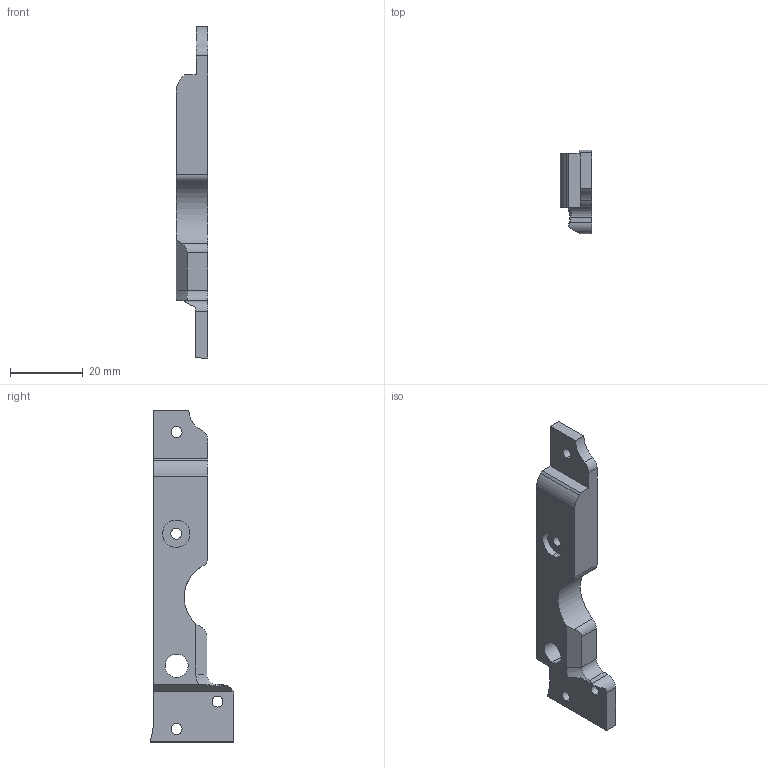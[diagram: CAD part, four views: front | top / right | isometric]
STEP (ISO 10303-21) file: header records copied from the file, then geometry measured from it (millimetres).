
FILE_DESCRIPTION (( 'STEP AP214' ), '1' );
FILE_NAME ('Thunderbolt_Buffer Tower_Split_Arm_Right.STEP', '2021-09-21T22:17:44', ( '' ), ( '' ), 'SwSTEP 2.0', 'SolidWorks 2020', '' );
FILE_SCHEMA (( 'AUTOMOTIVE_DESIGN' ));
Length unit declared in the file: millimetre
Products named in the file (1): Thunderbolt_Buffer Tower_Split_Arm_Right
Bounding box: 8.75 x 23.11 x 91.33 mm (x, y, z)
Volume: 8569.3 mm3; surface area: 4549.9 mm2
Topology: 1 solids, 1 shells, 39 faces, 107 edges, 71 vertices
Faces by surface type: cylinder 21, plane 17, cone 1
Entity records: 1325 total; most frequent: CARTESIAN_POINT 251, DIRECTION 222, ORIENTED_EDGE 214, EDGE_CURVE 107, AXIS2_PLACEMENT_3D 82, VERTEX_POINT 71, LINE 58, VECTOR 58
